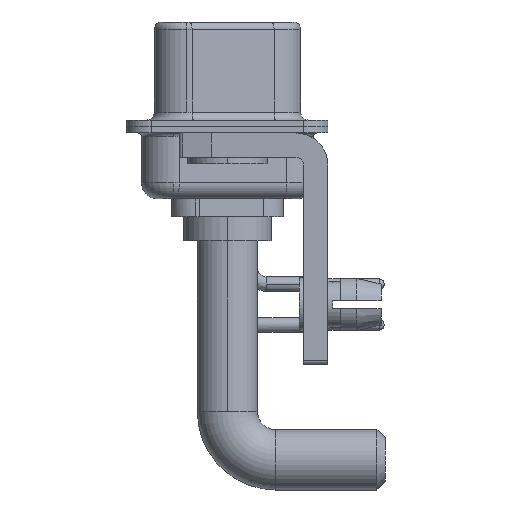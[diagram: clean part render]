
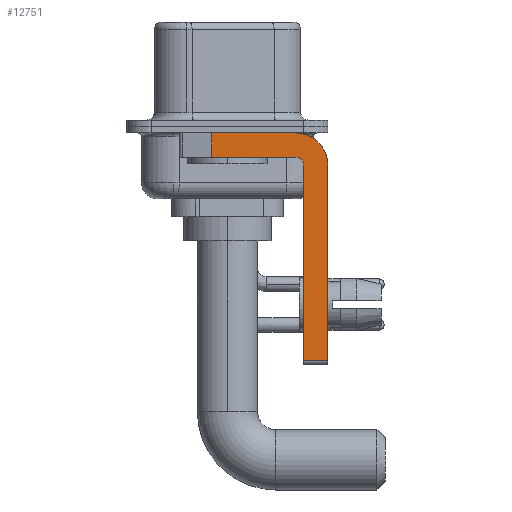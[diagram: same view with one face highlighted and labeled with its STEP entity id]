
A CAD part, left-side view. The second image highlights one B-rep face of the part: STEP entity #12751.
In plain terms, the highlighted planar face has unit normal (-1, 0, 0).
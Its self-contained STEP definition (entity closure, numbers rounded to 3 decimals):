
#64 = CARTESIAN_POINT ( 'NONE',  ( -2.9, -4.25, -2.4 ) ) ;
#828 = VERTEX_POINT ( 'NONE', #20214 ) ;
#834 = DIRECTION ( 'NONE',  ( 0., 0., 1. ) ) ;
#1290 = ORIENTED_EDGE ( 'NONE', *, *, #12025, .F. ) ;
#1372 = ORIENTED_EDGE ( 'NONE', *, *, #15902, .F. ) ;
#1470 = LINE ( 'NONE', #20220, #30448 ) ;
#1707 = VERTEX_POINT ( 'NONE', #23961 ) ;
#1878 = CARTESIAN_POINT ( 'NONE',  ( -2.9, 0.978, -0.4 ) ) ;
#2457 = DIRECTION ( 'NONE',  ( 0., 0., -1. ) ) ;
#2709 = DIRECTION ( 'NONE',  ( 1., 0., 0. ) ) ;
#3479 = DIRECTION ( 'NONE',  ( 1., 0., 0. ) ) ;
#3691 = ORIENTED_EDGE ( 'NONE', *, *, #21082, .F. ) ;
#5019 = VECTOR ( 'NONE', #26624, 1000. ) ;
#5486 = EDGE_LOOP ( 'NONE', ( #3691, #20763, #7560, #6082, #1290, #26742, #1372, #7103 ) ) ;
#5507 = CARTESIAN_POINT ( 'NONE',  ( -2.9, 3., -0.4 ) ) ;
#5608 = DIRECTION ( 'NONE',  ( 0., 1., 0. ) ) ;
#5778 = VERTEX_POINT ( 'NONE', #12014 ) ;
#6082 = ORIENTED_EDGE ( 'NONE', *, *, #20975, .F. ) ;
#7103 = ORIENTED_EDGE ( 'NONE', *, *, #22254, .F. ) ;
#7560 = ORIENTED_EDGE ( 'NONE', *, *, #8667, .F. ) ;
#8112 = CARTESIAN_POINT ( 'NONE',  ( -2.9, -4.25, -1.9 ) ) ;
#8178 = VECTOR ( 'NONE', #20740, 1000. ) ;
#8574 = EDGE_CURVE ( 'NONE', #16752, #8659, #14064, .T. ) ;
#8659 = VERTEX_POINT ( 'NONE', #17332 ) ;
#8667 = EDGE_CURVE ( 'NONE', #29258, #8659, #22023, .T. ) ;
#8710 = CARTESIAN_POINT ( 'NONE',  ( -2.9, -4.75, -14.8 ) ) ;
#9405 = VECTOR ( 'NONE', #14682, 1000. ) ;
#9946 = CARTESIAN_POINT ( 'NONE',  ( -2.9, -6.25, -2.4 ) ) ;
#10051 = DIRECTION ( 'NONE',  ( -1., 0., 0. ) ) ;
#10054 = CARTESIAN_POINT ( 'NONE',  ( -2.9, -4.25, -2.4 ) ) ;
#10605 = AXIS2_PLACEMENT_3D ( 'NONE', #10054, #3479, #12857 ) ;
#12014 = CARTESIAN_POINT ( 'NONE',  ( -2.9, -4.75, -14.55 ) ) ;
#12025 = EDGE_CURVE ( 'NONE', #5778, #20063, #15434, .T. ) ;
#12077 = CIRCLE ( 'NONE', #10605, 2. ) ;
#12751 = ADVANCED_FACE ( 'NONE', ( #16772 ), #22082, .F. ) ;
#12857 = DIRECTION ( 'NONE',  ( 0., 0., -1. ) ) ;
#13707 = AXIS2_PLACEMENT_3D ( 'NONE', #64, #2709, #26786 ) ;
#14064 = LINE ( 'NONE', #21255, #9405 ) ;
#14315 = VECTOR ( 'NONE', #2457, 1000. ) ;
#14682 = DIRECTION ( 'NONE',  ( 0., 0., -1. ) ) ;
#14958 = CARTESIAN_POINT ( 'NONE',  ( -2.9, -4.75, -2.4 ) ) ;
#15036 = CARTESIAN_POINT ( 'NONE',  ( -2.9, -4.25, -2.4 ) ) ;
#15434 = LINE ( 'NONE', #8710, #8178 ) ;
#15518 = CARTESIAN_POINT ( 'NONE',  ( -2.9, -4.25, -1.9 ) ) ;
#15902 = EDGE_CURVE ( 'NONE', #1707, #828, #26835, .T. ) ;
#16394 = VECTOR ( 'NONE', #5608, 1000. ) ;
#16752 = VERTEX_POINT ( 'NONE', #1878 ) ;
#16772 = FACE_OUTER_BOUND ( 'NONE', #5486, .T. ) ;
#17004 = CIRCLE ( 'NONE', #26508, 0.5 ) ;
#17332 = CARTESIAN_POINT ( 'NONE',  ( -2.9, 0.978, -1.9 ) ) ;
#17384 = LINE ( 'NONE', #5507, #5019 ) ;
#17927 = EDGE_CURVE ( 'NONE', #5778, #828, #1470, .T. ) ;
#20063 = VERTEX_POINT ( 'NONE', #14958 ) ;
#20214 = CARTESIAN_POINT ( 'NONE',  ( -2.9, -6.25, -14.55 ) ) ;
#20220 = CARTESIAN_POINT ( 'NONE',  ( -2.9, -4.25, -14.55 ) ) ;
#20740 = DIRECTION ( 'NONE',  ( 0., 0., 1. ) ) ;
#20763 = ORIENTED_EDGE ( 'NONE', *, *, #8574, .T. ) ;
#20826 = VERTEX_POINT ( 'NONE', #23646 ) ;
#20975 = EDGE_CURVE ( 'NONE', #20063, #29258, #17004, .T. ) ;
#21082 = EDGE_CURVE ( 'NONE', #16752, #20826, #17384, .T. ) ;
#21255 = CARTESIAN_POINT ( 'NONE',  ( -2.9, 0.978, -1.9 ) ) ;
#22023 = LINE ( 'NONE', #8112, #16394 ) ;
#22082 = PLANE ( 'NONE',  #13707 ) ;
#22254 = EDGE_CURVE ( 'NONE', #20826, #1707, #12077, .T. ) ;
#23646 = CARTESIAN_POINT ( 'NONE',  ( -2.9, -4.25, -0.4 ) ) ;
#23961 = CARTESIAN_POINT ( 'NONE',  ( -2.9, -6.25, -2.4 ) ) ;
#26508 = AXIS2_PLACEMENT_3D ( 'NONE', #15036, #10051, #834 ) ;
#26624 = DIRECTION ( 'NONE',  ( 0., -1., 0. ) ) ;
#26742 = ORIENTED_EDGE ( 'NONE', *, *, #17927, .T. ) ;
#26786 = DIRECTION ( 'NONE',  ( 0., 0., -1. ) ) ;
#26835 = LINE ( 'NONE', #9946, #14315 ) ;
#29258 = VERTEX_POINT ( 'NONE', #15518 ) ;
#29466 = DIRECTION ( 'NONE',  ( 0., -1., 0. ) ) ;
#30448 = VECTOR ( 'NONE', #29466, 1000. ) ;
